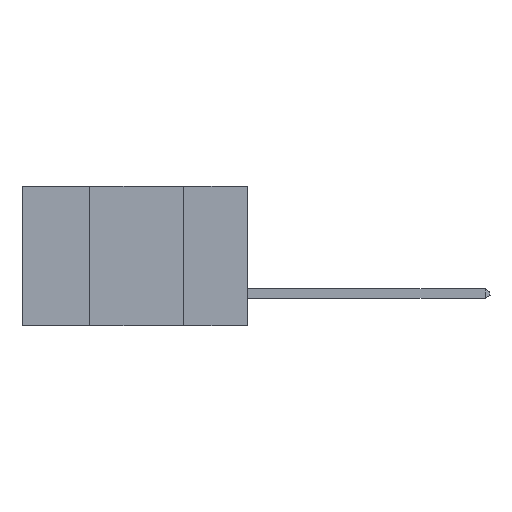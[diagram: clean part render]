
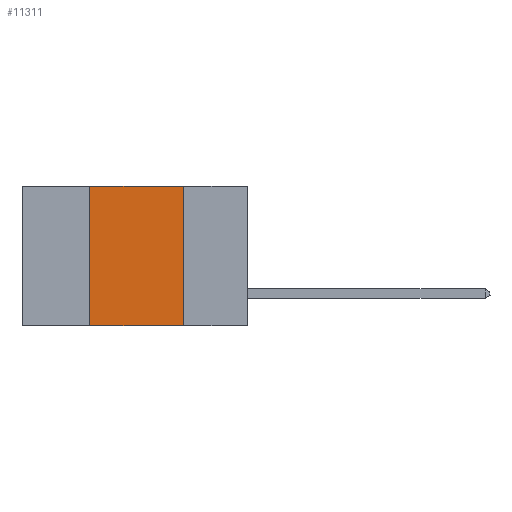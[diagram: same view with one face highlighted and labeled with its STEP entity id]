
A CAD part, left-side view. The second image highlights one B-rep face of the part: STEP entity #11311.
In plain terms, the highlighted planar face has unit normal (-1, 0, 0).
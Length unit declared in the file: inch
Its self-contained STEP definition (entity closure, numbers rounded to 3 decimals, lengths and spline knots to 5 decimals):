
#336 = ORIENTED_EDGE ( 'NONE', *, *, #1982, .T. ) ;
#883 = PLANE ( 'NONE',  #3245 ) ;
#1066 = DIRECTION ( 'NONE',  ( 0., 0., -1. ) ) ;
#1129 = DIRECTION ( 'NONE',  ( 0., -1., 0. ) ) ;
#1441 = EDGE_LOOP ( 'NONE', ( #18968, #17410, #13240, #336 ) ) ;
#1675 = LINE ( 'NONE', #17819, #14844 ) ;
#1704 = CARTESIAN_POINT ( 'NONE',  ( 0., 0.6, -0.37 ) ) ;
#1982 = EDGE_CURVE ( 'NONE', #1990, #11522, #11299, .T. ) ;
#1990 = VERTEX_POINT ( 'NONE', #4622 ) ;
#3245 = AXIS2_PLACEMENT_3D ( 'NONE', #17257, #9927, #1066 ) ;
#4150 = LINE ( 'NONE', #16004, #17023 ) ;
#4622 = CARTESIAN_POINT ( 'NONE',  ( 0., 0.42, -0.37 ) ) ;
#4892 = VERTEX_POINT ( 'NONE', #12481 ) ;
#5913 = EDGE_CURVE ( 'NONE', #18916, #11522, #1675, .T. ) ;
#6484 = CARTESIAN_POINT ( 'NONE',  ( 0., 0.17, -0.37 ) ) ;
#7515 = DIRECTION ( 'NONE',  ( 0., -1., 0. ) ) ;
#9386 = DIRECTION ( 'NONE',  ( 0., 0., 1. ) ) ;
#9927 = DIRECTION ( 'NONE',  ( 1., 0., 0. ) ) ;
#10501 = LINE ( 'NONE', #18214, #15824 ) ;
#10603 = VECTOR ( 'NONE', #7515, 39.37008 ) ;
#11299 = LINE ( 'NONE', #1704, #10603 ) ;
#11311 = ADVANCED_FACE ( 'NONE', ( #19068 ), #883, .F. ) ;
#11457 = CARTESIAN_POINT ( 'NONE',  ( 0., 0.17, 0. ) ) ;
#11522 = VERTEX_POINT ( 'NONE', #6484 ) ;
#12481 = CARTESIAN_POINT ( 'NONE',  ( 0., 0.42, 0. ) ) ;
#13240 = ORIENTED_EDGE ( 'NONE', *, *, #14058, .F. ) ;
#13527 = DIRECTION ( 'NONE',  ( 0., 0., -1. ) ) ;
#14058 = EDGE_CURVE ( 'NONE', #1990, #4892, #10501, .T. ) ;
#14844 = VECTOR ( 'NONE', #13527, 39.37008 ) ;
#15824 = VECTOR ( 'NONE', #9386, 39.37008 ) ;
#16004 = CARTESIAN_POINT ( 'NONE',  ( 0., 0.6, 0. ) ) ;
#17023 = VECTOR ( 'NONE', #1129, 39.37008 ) ;
#17257 = CARTESIAN_POINT ( 'NONE',  ( 0., 0.6, 0. ) ) ;
#17410 = ORIENTED_EDGE ( 'NONE', *, *, #18908, .F. ) ;
#17819 = CARTESIAN_POINT ( 'NONE',  ( 0., 0.17, 0. ) ) ;
#18214 = CARTESIAN_POINT ( 'NONE',  ( 0., 0.42, 0. ) ) ;
#18908 = EDGE_CURVE ( 'NONE', #4892, #18916, #4150, .T. ) ;
#18916 = VERTEX_POINT ( 'NONE', #11457 ) ;
#18968 = ORIENTED_EDGE ( 'NONE', *, *, #5913, .F. ) ;
#19068 = FACE_OUTER_BOUND ( 'NONE', #1441, .T. ) ;
